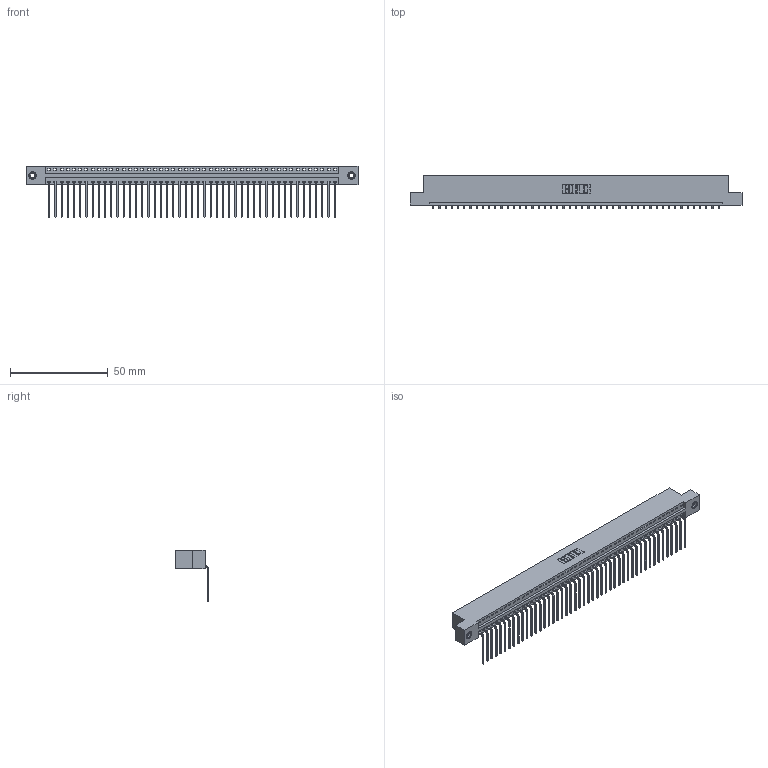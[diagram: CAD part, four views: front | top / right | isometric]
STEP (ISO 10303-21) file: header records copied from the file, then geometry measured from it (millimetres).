
FILE_DESCRIPTION (( 'STEP AP203' ), '1' );
FILE_NAME ('346-047-559-108.STEP', '2022-05-09T22:32:11', ( '' ), ( '' ), 'SwSTEP 2.0', 'SolidWorks 2020', '' );
FILE_SCHEMA (( 'CONFIG_CONTROL_DESIGN' ));
Length unit declared in the file: inch
Products named in the file (4): 345-250-001_345-250-003-102; 346-047-559-108; 345-292-001_558 559 Tail - 1; 346 Part_Flush Mounting Lugs - 0.156 Dia-TI
Assembly tree (50 placements, depth 2):
  346-047-559-108
    346 Part_Flush Mounting Lugs - 0.156 Dia-TI
    345-292-001_558 559 Tail - 1  x47
    345-250-001_345-250-003-102  x2
Bounding box: 169.8 x 17.08 x 26.16 mm (x, y, z)
Volume: 15744 mm3; surface area: 21486.6 mm2
Topology: 3 solids, 50 shells, 3002 faces, 8972 edges, 5895 vertices
Faces by surface type: plane 2082, cylinder 904, cone 12, torus 4
Entity records: 29766 total; most frequent: CARTESIAN_POINT 5084, ORIENTED_EDGE 5058, DIRECTION 4505, EDGE_CURVE 2529, VECTOR 2189, LINE 2189, VERTEX_POINT 1680, AXIS2_PLACEMENT_3D 1158
